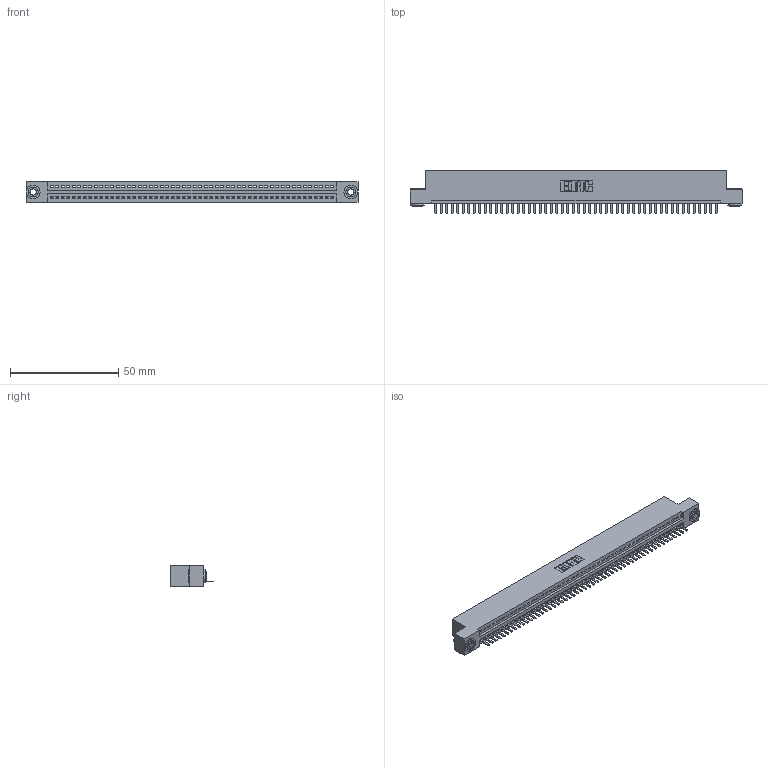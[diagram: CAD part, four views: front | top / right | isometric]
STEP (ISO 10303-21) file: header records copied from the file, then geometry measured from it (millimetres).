
FILE_DESCRIPTION (( 'STEP AP203' ), '1' );
FILE_NAME ('395-052-520-103.STEP', '2018-11-20T20:30:27', ( '' ), ( '' ), 'SwSTEP 2.0', 'SolidWorks 2016', '' );
FILE_SCHEMA (( 'CONFIG_CONTROL_DESIGN' ));
Length unit declared in the file: inch
Products named in the file (4): 345 Part_Flush Mounting Lugs - 0.156 Dia-TH; 395-052-520-103; 345-292-001_345-293-120; 345-250-002_345-250-002-102
Assembly tree (55 placements, depth 2):
  395-052-520-103
    345 Part_Flush Mounting Lugs - 0.156 Dia-TH
    345-292-001_345-293-120  x52
    345-250-002_345-250-002-102  x2
Bounding box: 153.29 x 19.68 x 9.4 mm (x, y, z)
Volume: 14511.3 mm3; surface area: 19145.2 mm2
Topology: 55 solids, 55 shells, 3388 faces, 9985 edges, 6514 vertices
Faces by surface type: plane 2274, cylinder 1106, cone 8
Entity records: 38554 total; most frequent: CARTESIAN_POINT 6667, ORIENTED_EDGE 6634, DIRECTION 5827, EDGE_CURVE 3317, LINE 2949, VECTOR 2949, VERTEX_POINT 2206, AXIS2_PLACEMENT_3D 1439
